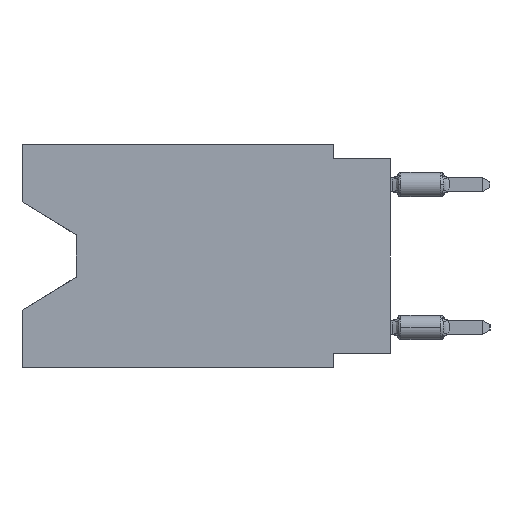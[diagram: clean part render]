
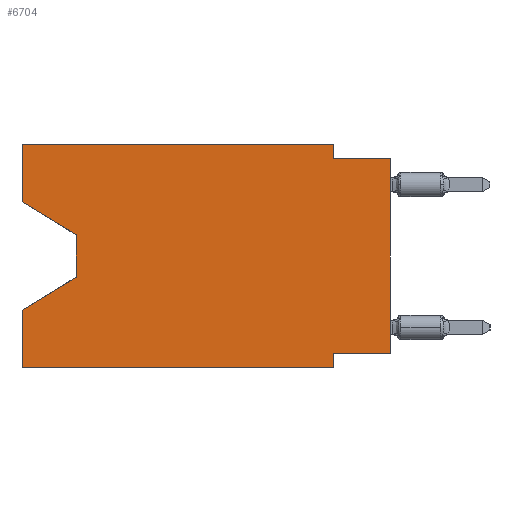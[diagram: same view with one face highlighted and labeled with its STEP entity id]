
A CAD part, left-side view. The second image highlights one B-rep face of the part: STEP entity #6704.
In plain terms, the highlighted planar face has unit normal (-1, 0, 0).
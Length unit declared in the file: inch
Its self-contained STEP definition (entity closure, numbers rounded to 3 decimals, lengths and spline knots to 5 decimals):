
#610 = VERTEX_POINT ( 'NONE', #21077 ) ;
#1010 = EDGE_CURVE ( 'NONE', #14191, #5006, #23110, .T. ) ;
#1138 = ORIENTED_EDGE ( 'NONE', *, *, #1243, .T. ) ;
#1243 = EDGE_CURVE ( 'NONE', #21215, #6378, #12073, .T. ) ;
#1244 = VECTOR ( 'NONE', #4401, 39.37008 ) ;
#2105 = VERTEX_POINT ( 'NONE', #10053 ) ;
#2362 = VECTOR ( 'NONE', #4805, 39.37008 ) ;
#3296 = CARTESIAN_POINT ( 'NONE',  ( 0., 0.55, -0.158 ) ) ;
#3435 = VECTOR ( 'NONE', #9886, 39.37008 ) ;
#3629 = LINE ( 'NONE', #12002, #21517 ) ;
#3699 = CARTESIAN_POINT ( 'NONE',  ( 0., 0.645, -0.39 ) ) ;
#3767 = DIRECTION ( 'NONE',  ( 0., -1., 0. ) ) ;
#3859 = CARTESIAN_POINT ( 'NONE',  ( 0., 0.55, -0.232 ) ) ;
#3890 = CARTESIAN_POINT ( 'NONE',  ( 0., 0.645, -0.39 ) ) ;
#4170 = CARTESIAN_POINT ( 'NONE',  ( 0., 0.1, -0.365 ) ) ;
#4401 = DIRECTION ( 'NONE',  ( 0., 1., 0. ) ) ;
#4562 = CARTESIAN_POINT ( 'NONE',  ( 0., 0.645, -0.10025 ) ) ;
#4805 = DIRECTION ( 'NONE',  ( 0., 0., -1. ) ) ;
#5006 = VERTEX_POINT ( 'NONE', #4170 ) ;
#5147 = LINE ( 'NONE', #15749, #17521 ) ;
#5490 = CARTESIAN_POINT ( 'NONE',  ( 0., 0.645, 0. ) ) ;
#6378 = VERTEX_POINT ( 'NONE', #10336 ) ;
#6647 = VERTEX_POINT ( 'NONE', #3296 ) ;
#6704 = ADVANCED_FACE ( 'NONE', ( #7560 ), #15959, .F. ) ;
#6850 = CARTESIAN_POINT ( 'NONE',  ( 0., 0.1, 0. ) ) ;
#6973 = CARTESIAN_POINT ( 'NONE',  ( 0., 0.1, -0.39 ) ) ;
#7017 = EDGE_CURVE ( 'NONE', #5006, #15843, #15648, .T. ) ;
#7393 = LINE ( 'NONE', #20196, #17488 ) ;
#7560 = FACE_OUTER_BOUND ( 'NONE', #12715, .T. ) ;
#8021 = LINE ( 'NONE', #3890, #25634 ) ;
#8243 = LINE ( 'NONE', #24782, #13476 ) ;
#8425 = CARTESIAN_POINT ( 'NONE',  ( 0., 0., -0.365 ) ) ;
#8666 = ORIENTED_EDGE ( 'NONE', *, *, #13534, .T. ) ;
#8812 = DIRECTION ( 'NONE',  ( 0., -1., 0. ) ) ;
#9135 = EDGE_CURVE ( 'NONE', #22419, #6647, #8243, .T. ) ;
#9368 = VECTOR ( 'NONE', #8812, 39.37008 ) ;
#9441 = EDGE_CURVE ( 'NONE', #10036, #23462, #11650, .T. ) ;
#9886 = DIRECTION ( 'NONE',  ( 0., 0.855, -0.519 ) ) ;
#10036 = VERTEX_POINT ( 'NONE', #21048 ) ;
#10053 = CARTESIAN_POINT ( 'NONE',  ( 0., 0., -0.025 ) ) ;
#10336 = CARTESIAN_POINT ( 'NONE',  ( 0., 0.645, -0.28975 ) ) ;
#11208 = CARTESIAN_POINT ( 'NONE',  ( 0., 0.1, 0. ) ) ;
#11392 = VECTOR ( 'NONE', #15530, 39.37008 ) ;
#11650 = LINE ( 'NONE', #17998, #25788 ) ;
#12002 = CARTESIAN_POINT ( 'NONE',  ( 0., 0.645, 0. ) ) ;
#12073 = LINE ( 'NONE', #18139, #3435 ) ;
#12144 = DIRECTION ( 'NONE',  ( 0., 0., 1. ) ) ;
#12715 = EDGE_LOOP ( 'NONE', ( #25629, #8666, #1138, #16075, #25968, #22397, #26180, #26738, #16440, #22545, #17080, #16255 ) ) ;
#12936 = LINE ( 'NONE', #15792, #9368 ) ;
#13476 = VECTOR ( 'NONE', #18440, 39.37008 ) ;
#13534 = EDGE_CURVE ( 'NONE', #6647, #21215, #5147, .T. ) ;
#14121 = EDGE_CURVE ( 'NONE', #22419, #10036, #3629, .T. ) ;
#14191 = VERTEX_POINT ( 'NONE', #8425 ) ;
#15530 = DIRECTION ( 'NONE',  ( 0., 0., 1. ) ) ;
#15648 = LINE ( 'NONE', #6973, #24165 ) ;
#15749 = CARTESIAN_POINT ( 'NONE',  ( 0., 0.55, -0.158 ) ) ;
#15792 = CARTESIAN_POINT ( 'NONE',  ( 0., 0., -0.025 ) ) ;
#15843 = VERTEX_POINT ( 'NONE', #21344 ) ;
#15959 = PLANE ( 'NONE',  #23237 ) ;
#16024 = DIRECTION ( 'NONE',  ( 0., 0., -1. ) ) ;
#16075 = ORIENTED_EDGE ( 'NONE', *, *, #25896, .F. ) ;
#16255 = ORIENTED_EDGE ( 'NONE', *, *, #14121, .F. ) ;
#16440 = ORIENTED_EDGE ( 'NONE', *, *, #18477, .F. ) ;
#17080 = ORIENTED_EDGE ( 'NONE', *, *, #9441, .F. ) ;
#17330 = LINE ( 'NONE', #6850, #2362 ) ;
#17488 = VECTOR ( 'NONE', #24337, 39.37008 ) ;
#17521 = VECTOR ( 'NONE', #16024, 39.37008 ) ;
#17598 = CARTESIAN_POINT ( 'NONE',  ( 0., 0.645, 0. ) ) ;
#17998 = CARTESIAN_POINT ( 'NONE',  ( 0., 0.645, 0. ) ) ;
#18139 = CARTESIAN_POINT ( 'NONE',  ( 0., 0.55, -0.232 ) ) ;
#18440 = DIRECTION ( 'NONE',  ( 0., -0.855, -0.519 ) ) ;
#18477 = EDGE_CURVE ( 'NONE', #610, #2105, #12936, .T. ) ;
#20196 = CARTESIAN_POINT ( 'NONE',  ( 0., 0., 0. ) ) ;
#20225 = EDGE_CURVE ( 'NONE', #23462, #610, #17330, .T. ) ;
#20246 = VERTEX_POINT ( 'NONE', #3699 ) ;
#20747 = EDGE_CURVE ( 'NONE', #20246, #15843, #8021, .T. ) ;
#21048 = CARTESIAN_POINT ( 'NONE',  ( 0., 0.645, 0. ) ) ;
#21077 = CARTESIAN_POINT ( 'NONE',  ( 0., 0.1, -0.025 ) ) ;
#21215 = VERTEX_POINT ( 'NONE', #3859 ) ;
#21344 = CARTESIAN_POINT ( 'NONE',  ( 0., 0.1, -0.39 ) ) ;
#21517 = VECTOR ( 'NONE', #12144, 39.37008 ) ;
#21744 = DIRECTION ( 'NONE',  ( 0., 0., -1. ) ) ;
#22397 = ORIENTED_EDGE ( 'NONE', *, *, #7017, .F. ) ;
#22419 = VERTEX_POINT ( 'NONE', #4562 ) ;
#22545 = ORIENTED_EDGE ( 'NONE', *, *, #20225, .F. ) ;
#23110 = LINE ( 'NONE', #27118, #1244 ) ;
#23237 = AXIS2_PLACEMENT_3D ( 'NONE', #5490, #24488, #21744 ) ;
#23462 = VERTEX_POINT ( 'NONE', #11208 ) ;
#24053 = DIRECTION ( 'NONE',  ( 0., -1., 0. ) ) ;
#24155 = EDGE_CURVE ( 'NONE', #14191, #2105, #7393, .T. ) ;
#24165 = VECTOR ( 'NONE', #26239, 39.37008 ) ;
#24337 = DIRECTION ( 'NONE',  ( 0., 0., 1. ) ) ;
#24345 = LINE ( 'NONE', #17598, #11392 ) ;
#24488 = DIRECTION ( 'NONE',  ( 1., 0., 0. ) ) ;
#24782 = CARTESIAN_POINT ( 'NONE',  ( 0., 0.645, -0.10025 ) ) ;
#25629 = ORIENTED_EDGE ( 'NONE', *, *, #9135, .T. ) ;
#25634 = VECTOR ( 'NONE', #3767, 39.37008 ) ;
#25788 = VECTOR ( 'NONE', #24053, 39.37008 ) ;
#25896 = EDGE_CURVE ( 'NONE', #20246, #6378, #24345, .T. ) ;
#25968 = ORIENTED_EDGE ( 'NONE', *, *, #20747, .T. ) ;
#26180 = ORIENTED_EDGE ( 'NONE', *, *, #1010, .F. ) ;
#26239 = DIRECTION ( 'NONE',  ( 0., 0., -1. ) ) ;
#26738 = ORIENTED_EDGE ( 'NONE', *, *, #24155, .T. ) ;
#27118 = CARTESIAN_POINT ( 'NONE',  ( 0., 0., -0.365 ) ) ;
